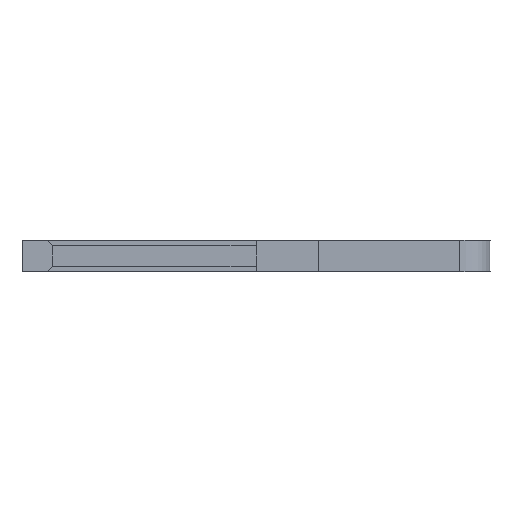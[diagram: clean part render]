
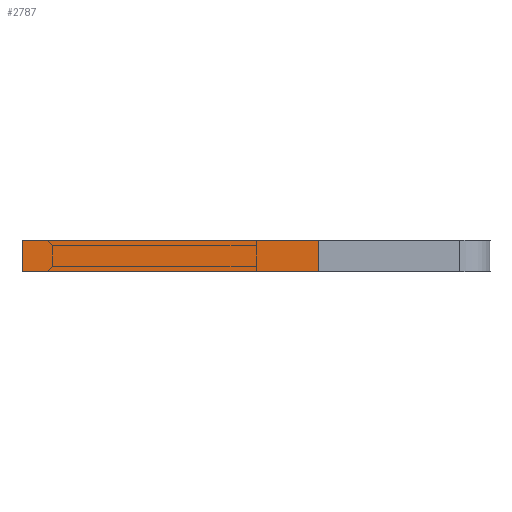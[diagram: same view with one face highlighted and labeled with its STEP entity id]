
A CAD part, left-side view. The second image highlights one B-rep face of the part: STEP entity #2787.
In plain terms, the highlighted face is planar.
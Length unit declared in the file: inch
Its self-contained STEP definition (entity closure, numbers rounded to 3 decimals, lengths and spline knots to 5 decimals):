
#42 = EDGE_CURVE ( 'NONE', #1589, #3063, #1323, .T. ) ;
#156 = DIRECTION ( 'NONE',  ( 0., 0., 1. ) ) ;
#262 = EDGE_CURVE ( 'NONE', #4013, #1484, #4259, .T. ) ;
#486 = ORIENTED_EDGE ( 'NONE', *, *, #262, .T. ) ;
#582 = LINE ( 'NONE', #2562, #2239 ) ;
#764 = CARTESIAN_POINT ( 'NONE',  ( 0.01, 0.15, -0.04 ) ) ;
#791 = CARTESIAN_POINT ( 'NONE',  ( 0.01, 0.15, -0.04 ) ) ;
#966 = CARTESIAN_POINT ( 'NONE',  ( -0.01, 0.15, -0.04 ) ) ;
#1171 = EDGE_CURVE ( 'NONE', #3063, #1484, #3056, .T. ) ;
#1220 = VECTOR ( 'NONE', #1513, 39.37008 ) ;
#1285 = ORIENTED_EDGE ( 'NONE', *, *, #1171, .F. ) ;
#1323 = LINE ( 'NONE', #764, #3529 ) ;
#1465 = PLANE ( 'NONE',  #3871 ) ;
#1484 = VERTEX_POINT ( 'NONE', #966 ) ;
#1513 = DIRECTION ( 'NONE',  ( 0., 1., 0. ) ) ;
#1589 = VERTEX_POINT ( 'NONE', #2297 ) ;
#1632 = DIRECTION ( 'NONE',  ( -1., 0., 0. ) ) ;
#1816 = EDGE_LOOP ( 'NONE', ( #486, #1285, #3596, #3651 ) ) ;
#2142 = VECTOR ( 'NONE', #1632, 39.37008 ) ;
#2239 = VECTOR ( 'NONE', #2604, 39.37008 ) ;
#2297 = CARTESIAN_POINT ( 'NONE',  ( 0.01, -0.04, -0.04 ) ) ;
#2499 = CARTESIAN_POINT ( 'NONE',  ( 0.01, 0.15, -0.04 ) ) ;
#2562 = CARTESIAN_POINT ( 'NONE',  ( 0.01, -0.04, -0.04 ) ) ;
#2604 = DIRECTION ( 'NONE',  ( -1., 0., 0. ) ) ;
#2787 = ADVANCED_FACE ( 'NONE', ( #3413 ), #1465, .F. ) ;
#2824 = CARTESIAN_POINT ( 'NONE',  ( -0.01, 0.15, -0.04 ) ) ;
#3056 = LINE ( 'NONE', #3304, #2142 ) ;
#3063 = VERTEX_POINT ( 'NONE', #791 ) ;
#3237 = DIRECTION ( 'NONE',  ( 1., 0., 0. ) ) ;
#3304 = CARTESIAN_POINT ( 'NONE',  ( 0.01, 0.15, -0.04 ) ) ;
#3413 = FACE_OUTER_BOUND ( 'NONE', #1816, .T. ) ;
#3529 = VECTOR ( 'NONE', #4201, 39.37008 ) ;
#3596 = ORIENTED_EDGE ( 'NONE', *, *, #42, .F. ) ;
#3603 = CARTESIAN_POINT ( 'NONE',  ( -0.01, -0.04, -0.04 ) ) ;
#3651 = ORIENTED_EDGE ( 'NONE', *, *, #3809, .T. ) ;
#3809 = EDGE_CURVE ( 'NONE', #1589, #4013, #582, .T. ) ;
#3871 = AXIS2_PLACEMENT_3D ( 'NONE', #2499, #156, #3237 ) ;
#4013 = VERTEX_POINT ( 'NONE', #3603 ) ;
#4201 = DIRECTION ( 'NONE',  ( 0., 1., 0. ) ) ;
#4259 = LINE ( 'NONE', #2824, #1220 ) ;
